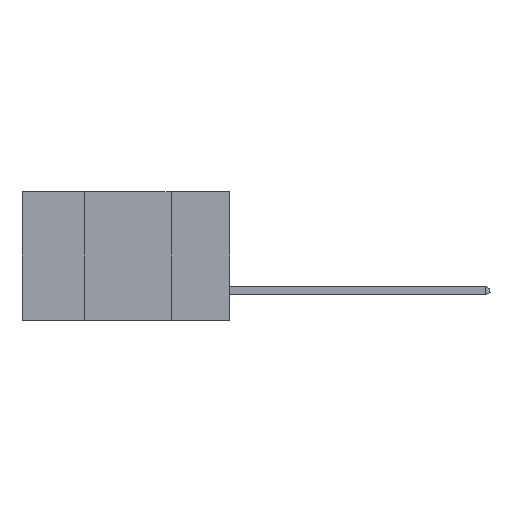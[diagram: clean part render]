
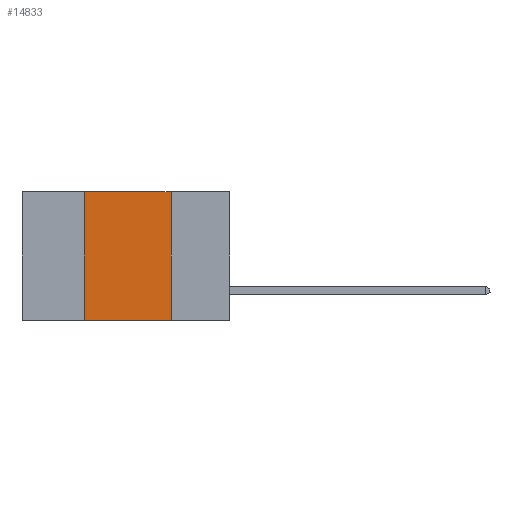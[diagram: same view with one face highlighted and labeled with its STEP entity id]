
A CAD part, left-side view. The second image highlights one B-rep face of the part: STEP entity #14833.
In plain terms, the highlighted planar face has unit normal (-1, 0, 0).
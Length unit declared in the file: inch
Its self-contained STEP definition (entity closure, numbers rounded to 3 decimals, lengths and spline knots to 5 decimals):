
#9 = VERTEX_POINT ( 'NONE', #11271 ) ;
#2682 = LINE ( 'NONE', #17558, #14959 ) ;
#3114 = DIRECTION ( 'NONE',  ( 0., -1., 0. ) ) ;
#3194 = EDGE_CURVE ( 'NONE', #17496, #9, #6119, .T. ) ;
#4179 = DIRECTION ( 'NONE',  ( 0., 0., -1. ) ) ;
#5628 = DIRECTION ( 'NONE',  ( 1., 0., 0. ) ) ;
#6119 = LINE ( 'NONE', #9434, #14004 ) ;
#6539 = CARTESIAN_POINT ( 'NONE',  ( 0., 0.6, -0.37 ) ) ;
#6815 = DIRECTION ( 'NONE',  ( 0., 0., -1. ) ) ;
#7124 = CARTESIAN_POINT ( 'NONE',  ( 0., 0.6, 0. ) ) ;
#7827 = EDGE_CURVE ( 'NONE', #17496, #14748, #9776, .T. ) ;
#8827 = AXIS2_PLACEMENT_3D ( 'NONE', #7124, #5628, #4179 ) ;
#9400 = VECTOR ( 'NONE', #3114, 39.37008 ) ;
#9434 = CARTESIAN_POINT ( 'NONE',  ( 0., 0.42, 0. ) ) ;
#9718 = DIRECTION ( 'NONE',  ( 0., 0., 1. ) ) ;
#9776 = LINE ( 'NONE', #6539, #13958 ) ;
#10034 = EDGE_CURVE ( 'NONE', #11487, #14748, #2682, .T. ) ;
#10383 = LINE ( 'NONE', #12584, #9400 ) ;
#11009 = ORIENTED_EDGE ( 'NONE', *, *, #10034, .F. ) ;
#11271 = CARTESIAN_POINT ( 'NONE',  ( 0., 0.42, 0. ) ) ;
#11487 = VERTEX_POINT ( 'NONE', #15872 ) ;
#12584 = CARTESIAN_POINT ( 'NONE',  ( 0., 0.6, 0. ) ) ;
#12989 = CARTESIAN_POINT ( 'NONE',  ( 0., 0.17, -0.37 ) ) ;
#13127 = ORIENTED_EDGE ( 'NONE', *, *, #7827, .T. ) ;
#13595 = PLANE ( 'NONE',  #8827 ) ;
#13958 = VECTOR ( 'NONE', #17562, 39.37008 ) ;
#14004 = VECTOR ( 'NONE', #9718, 39.37008 ) ;
#14748 = VERTEX_POINT ( 'NONE', #12989 ) ;
#14833 = ADVANCED_FACE ( 'NONE', ( #20267 ), #13595, .F. ) ;
#14959 = VECTOR ( 'NONE', #6815, 39.37008 ) ;
#15872 = CARTESIAN_POINT ( 'NONE',  ( 0., 0.17, 0. ) ) ;
#16472 = CARTESIAN_POINT ( 'NONE',  ( 0., 0.42, -0.37 ) ) ;
#17496 = VERTEX_POINT ( 'NONE', #16472 ) ;
#17558 = CARTESIAN_POINT ( 'NONE',  ( 0., 0.17, 0. ) ) ;
#17562 = DIRECTION ( 'NONE',  ( 0., -1., 0. ) ) ;
#18537 = ORIENTED_EDGE ( 'NONE', *, *, #3194, .F. ) ;
#19176 = EDGE_CURVE ( 'NONE', #9, #11487, #10383, .T. ) ;
#19591 = ORIENTED_EDGE ( 'NONE', *, *, #19176, .F. ) ;
#19740 = EDGE_LOOP ( 'NONE', ( #11009, #19591, #18537, #13127 ) ) ;
#20267 = FACE_OUTER_BOUND ( 'NONE', #19740, .T. ) ;
